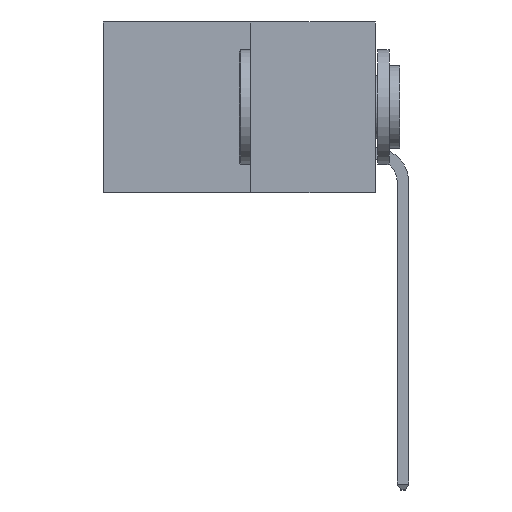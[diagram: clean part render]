
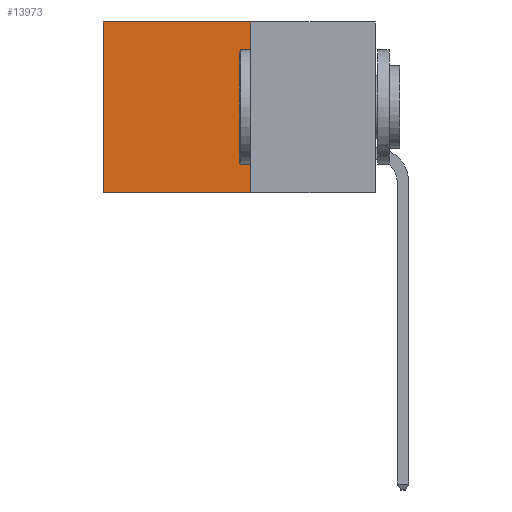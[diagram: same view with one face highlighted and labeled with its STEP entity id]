
A CAD part, left-side view. The second image highlights one B-rep face of the part: STEP entity #13973.
In plain terms, the highlighted planar face has unit normal (-1, 0, 0).
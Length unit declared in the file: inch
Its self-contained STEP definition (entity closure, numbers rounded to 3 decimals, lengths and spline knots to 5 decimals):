
#1063 = CARTESIAN_POINT ( 'NONE',  ( 0.277, 0.59, -0.37 ) ) ;
#1188 = EDGE_CURVE ( 'NONE', #2442, #2263, #13059, .T. ) ;
#2263 = VERTEX_POINT ( 'NONE', #1063 ) ;
#2442 = VERTEX_POINT ( 'NONE', #3881 ) ;
#3881 = CARTESIAN_POINT ( 'NONE',  ( 0.277, 0.59, 0. ) ) ;
#3941 = DIRECTION ( 'NONE',  ( 0., 1., 0. ) ) ;
#4180 = VECTOR ( 'NONE', #3941, 39.37008 ) ;
#4189 = EDGE_CURVE ( 'NONE', #9811, #17202, #14014, .T. ) ;
#6540 = EDGE_LOOP ( 'NONE', ( #12439, #24167, #20859, #28142 ) ) ;
#6776 = VECTOR ( 'NONE', #18986, 39.37008 ) ;
#6816 = PLANE ( 'NONE',  #23127 ) ;
#8268 = LINE ( 'NONE', #27549, #26113 ) ;
#8403 = FACE_OUTER_BOUND ( 'NONE', #6540, .T. ) ;
#9368 = EDGE_CURVE ( 'NONE', #9811, #2442, #8268, .T. ) ;
#9811 = VERTEX_POINT ( 'NONE', #15325 ) ;
#10142 = EDGE_CURVE ( 'NONE', #17202, #2263, #16816, .T. ) ;
#11551 = CARTESIAN_POINT ( 'NONE',  ( 0.277, 0.27, -0.37 ) ) ;
#12439 = ORIENTED_EDGE ( 'NONE', *, *, #1188, .T. ) ;
#13059 = LINE ( 'NONE', #29384, #6776 ) ;
#13286 = VECTOR ( 'NONE', #19565, 39.37008 ) ;
#13962 = DIRECTION ( 'NONE',  ( 1., 0., 0. ) ) ;
#13973 = ADVANCED_FACE ( 'NONE', ( #8403 ), #6816, .F. ) ;
#14014 = LINE ( 'NONE', #19246, #13286 ) ;
#15325 = CARTESIAN_POINT ( 'NONE',  ( 0.277, 0.27, 0. ) ) ;
#15775 = CARTESIAN_POINT ( 'NONE',  ( 0.277, 0.27, -0.37 ) ) ;
#16816 = LINE ( 'NONE', #15775, #4180 ) ;
#17202 = VERTEX_POINT ( 'NONE', #27484 ) ;
#18986 = DIRECTION ( 'NONE',  ( 0., 0., -1. ) ) ;
#19246 = CARTESIAN_POINT ( 'NONE',  ( 0.277, 0.27, -0.37 ) ) ;
#19565 = DIRECTION ( 'NONE',  ( 0., 0., -1. ) ) ;
#20859 = ORIENTED_EDGE ( 'NONE', *, *, #4189, .F. ) ;
#23127 = AXIS2_PLACEMENT_3D ( 'NONE', #11551, #13962, #30007 ) ;
#24167 = ORIENTED_EDGE ( 'NONE', *, *, #10142, .F. ) ;
#26113 = VECTOR ( 'NONE', #29826, 39.37008 ) ;
#27484 = CARTESIAN_POINT ( 'NONE',  ( 0.277, 0.27, -0.37 ) ) ;
#27549 = CARTESIAN_POINT ( 'NONE',  ( 0.277, 0.27, 0. ) ) ;
#28142 = ORIENTED_EDGE ( 'NONE', *, *, #9368, .T. ) ;
#29384 = CARTESIAN_POINT ( 'NONE',  ( 0.277, 0.59, -0.37 ) ) ;
#29826 = DIRECTION ( 'NONE',  ( 0., 1., 0. ) ) ;
#30007 = DIRECTION ( 'NONE',  ( 0., 0., -1. ) ) ;
